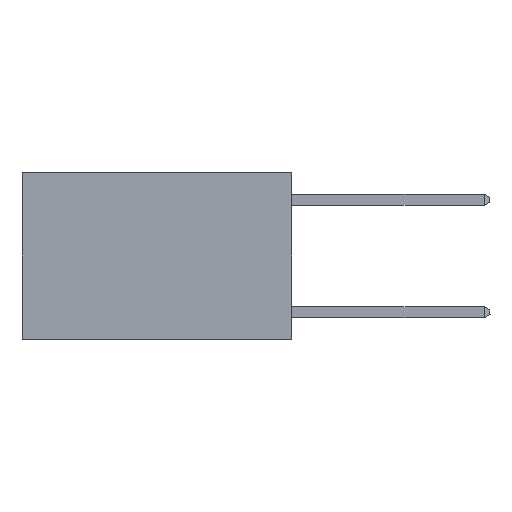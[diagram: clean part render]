
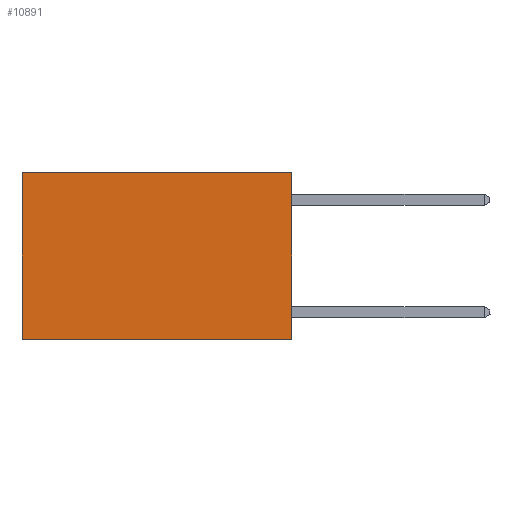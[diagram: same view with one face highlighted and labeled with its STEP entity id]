
A CAD part, left-side view. The second image highlights one B-rep face of the part: STEP entity #10891.
In plain terms, the highlighted planar face has unit normal (-1, 0, 0).
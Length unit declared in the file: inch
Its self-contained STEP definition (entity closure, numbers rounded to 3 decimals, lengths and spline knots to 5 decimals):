
#733 = EDGE_CURVE ( 'NONE', #11677, #21101, #21314, .T. ) ;
#1262 = EDGE_CURVE ( 'NONE', #10036, #21101, #6755, .T. ) ;
#3682 = ORIENTED_EDGE ( 'NONE', *, *, #733, .F. ) ;
#4061 = CARTESIAN_POINT ( 'NONE',  ( 0.2625, 0., 0. ) ) ;
#4135 = DIRECTION ( 'NONE',  ( 0., 1., 0. ) ) ;
#5044 = LINE ( 'NONE', #19450, #18993 ) ;
#5392 = DIRECTION ( 'NONE',  ( 0., 0., -1. ) ) ;
#6082 = EDGE_CURVE ( 'NONE', #7585, #10036, #17810, .T. ) ;
#6755 = LINE ( 'NONE', #16605, #15309 ) ;
#6991 = PLANE ( 'NONE',  #20816 ) ;
#7585 = VERTEX_POINT ( 'NONE', #11994 ) ;
#8462 = EDGE_LOOP ( 'NONE', ( #20243, #3682, #9742, #14922 ) ) ;
#9742 = ORIENTED_EDGE ( 'NONE', *, *, #12139, .F. ) ;
#10036 = VERTEX_POINT ( 'NONE', #22466 ) ;
#10805 = CARTESIAN_POINT ( 'NONE',  ( 0.2625, 0., 0. ) ) ;
#10891 = ADVANCED_FACE ( 'NONE', ( #21046 ), #6991, .F. ) ;
#11595 = VECTOR ( 'NONE', #17748, 39.37008 ) ;
#11672 = DIRECTION ( 'NONE',  ( 1., 0., 0. ) ) ;
#11677 = VERTEX_POINT ( 'NONE', #16532 ) ;
#11757 = CARTESIAN_POINT ( 'NONE',  ( 0.2625, 0.6, -0.37 ) ) ;
#11994 = CARTESIAN_POINT ( 'NONE',  ( 0.2625, 0., 0. ) ) ;
#12139 = EDGE_CURVE ( 'NONE', #7585, #11677, #5044, .T. ) ;
#12614 = DIRECTION ( 'NONE',  ( 0., 0., -1. ) ) ;
#13940 = DIRECTION ( 'NONE',  ( 0., 0., -1. ) ) ;
#14922 = ORIENTED_EDGE ( 'NONE', *, *, #6082, .T. ) ;
#15309 = VECTOR ( 'NONE', #5392, 39.37008 ) ;
#16532 = CARTESIAN_POINT ( 'NONE',  ( 0.2625, 0., -0.37 ) ) ;
#16605 = CARTESIAN_POINT ( 'NONE',  ( 0.2625, 0.6, 0. ) ) ;
#17748 = DIRECTION ( 'NONE',  ( 0., 1., 0. ) ) ;
#17810 = LINE ( 'NONE', #4061, #22094 ) ;
#18559 = CARTESIAN_POINT ( 'NONE',  ( 0.2625, 0., -0.37 ) ) ;
#18993 = VECTOR ( 'NONE', #13940, 39.37008 ) ;
#19450 = CARTESIAN_POINT ( 'NONE',  ( 0.2625, 0., 0. ) ) ;
#20243 = ORIENTED_EDGE ( 'NONE', *, *, #1262, .T. ) ;
#20816 = AXIS2_PLACEMENT_3D ( 'NONE', #10805, #11672, #12614 ) ;
#21046 = FACE_OUTER_BOUND ( 'NONE', #8462, .T. ) ;
#21101 = VERTEX_POINT ( 'NONE', #11757 ) ;
#21314 = LINE ( 'NONE', #18559, #11595 ) ;
#22094 = VECTOR ( 'NONE', #4135, 39.37008 ) ;
#22466 = CARTESIAN_POINT ( 'NONE',  ( 0.2625, 0.6, 0. ) ) ;
